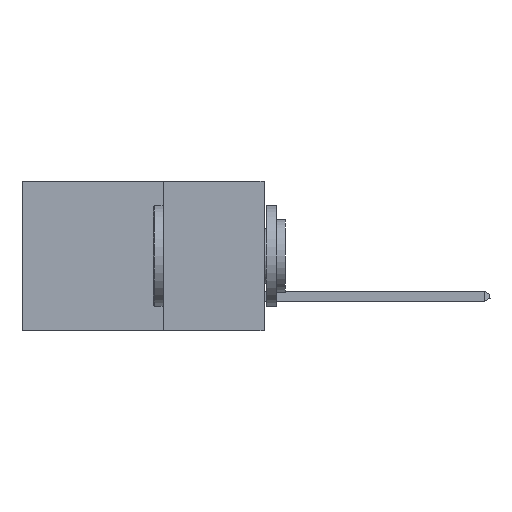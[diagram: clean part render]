
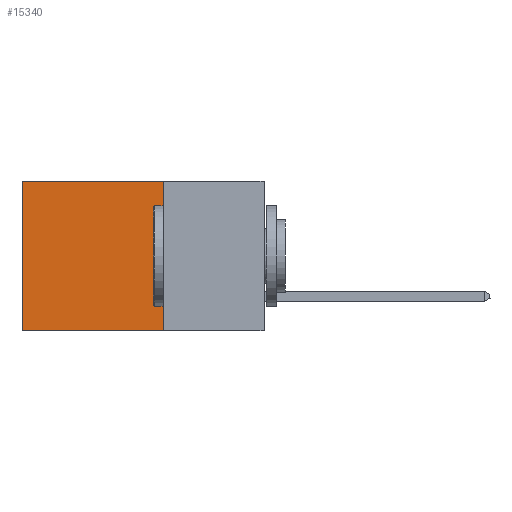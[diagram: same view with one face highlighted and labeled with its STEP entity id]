
A CAD part, left-side view. The second image highlights one B-rep face of the part: STEP entity #15340.
In plain terms, the highlighted planar face has unit normal (-1, 0, 0).
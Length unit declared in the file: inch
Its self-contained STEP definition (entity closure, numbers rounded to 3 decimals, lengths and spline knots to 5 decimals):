
#402 = DIRECTION ( 'NONE',  ( 0., 1., 0. ) ) ;
#1496 = CARTESIAN_POINT ( 'NONE',  ( 0.298, 0.25, -0.37 ) ) ;
#1746 = FACE_OUTER_BOUND ( 'NONE', #12357, .T. ) ;
#1809 = VECTOR ( 'NONE', #5956, 39.37008 ) ;
#2117 = AXIS2_PLACEMENT_3D ( 'NONE', #12856, #19074, #8314 ) ;
#2156 = VERTEX_POINT ( 'NONE', #8595 ) ;
#2240 = VERTEX_POINT ( 'NONE', #13147 ) ;
#2592 = CARTESIAN_POINT ( 'NONE',  ( 0.298, 0.25, 0. ) ) ;
#3579 = VECTOR ( 'NONE', #3785, 39.37008 ) ;
#3785 = DIRECTION ( 'NONE',  ( 0., 0., -1. ) ) ;
#4162 = LINE ( 'NONE', #7269, #1809 ) ;
#4272 = EDGE_CURVE ( 'NONE', #16687, #2240, #4162, .T. ) ;
#4311 = LINE ( 'NONE', #1496, #11422 ) ;
#4328 = DIRECTION ( 'NONE',  ( 0., 1., 0. ) ) ;
#5956 = DIRECTION ( 'NONE',  ( 0., 0., -1. ) ) ;
#6234 = CARTESIAN_POINT ( 'NONE',  ( 0.298, 0.25, 0. ) ) ;
#7269 = CARTESIAN_POINT ( 'NONE',  ( 0.298, 0.25, 0. ) ) ;
#7559 = LINE ( 'NONE', #15735, #3579 ) ;
#8140 = ORIENTED_EDGE ( 'NONE', *, *, #10493, .T. ) ;
#8314 = DIRECTION ( 'NONE',  ( 0., 0., -1. ) ) ;
#8437 = PLANE ( 'NONE',  #2117 ) ;
#8595 = CARTESIAN_POINT ( 'NONE',  ( 0.298, 0.6, 0. ) ) ;
#8995 = VECTOR ( 'NONE', #402, 39.37008 ) ;
#10493 = EDGE_CURVE ( 'NONE', #16687, #2156, #17109, .T. ) ;
#10939 = ORIENTED_EDGE ( 'NONE', *, *, #4272, .F. ) ;
#11422 = VECTOR ( 'NONE', #4328, 39.37008 ) ;
#12135 = CARTESIAN_POINT ( 'NONE',  ( 0.298, 0.6, -0.37 ) ) ;
#12357 = EDGE_LOOP ( 'NONE', ( #15359, #16311, #10939, #8140 ) ) ;
#12856 = CARTESIAN_POINT ( 'NONE',  ( 0.298, 0.25, 0. ) ) ;
#13147 = CARTESIAN_POINT ( 'NONE',  ( 0.298, 0.25, -0.37 ) ) ;
#15340 = ADVANCED_FACE ( 'NONE', ( #1746 ), #8437, .F. ) ;
#15359 = ORIENTED_EDGE ( 'NONE', *, *, #16651, .T. ) ;
#15735 = CARTESIAN_POINT ( 'NONE',  ( 0.298, 0.6, 0. ) ) ;
#16311 = ORIENTED_EDGE ( 'NONE', *, *, #18493, .F. ) ;
#16651 = EDGE_CURVE ( 'NONE', #2156, #19116, #7559, .T. ) ;
#16687 = VERTEX_POINT ( 'NONE', #2592 ) ;
#17109 = LINE ( 'NONE', #6234, #8995 ) ;
#18493 = EDGE_CURVE ( 'NONE', #2240, #19116, #4311, .T. ) ;
#19074 = DIRECTION ( 'NONE',  ( 1., 0., 0. ) ) ;
#19116 = VERTEX_POINT ( 'NONE', #12135 ) ;
